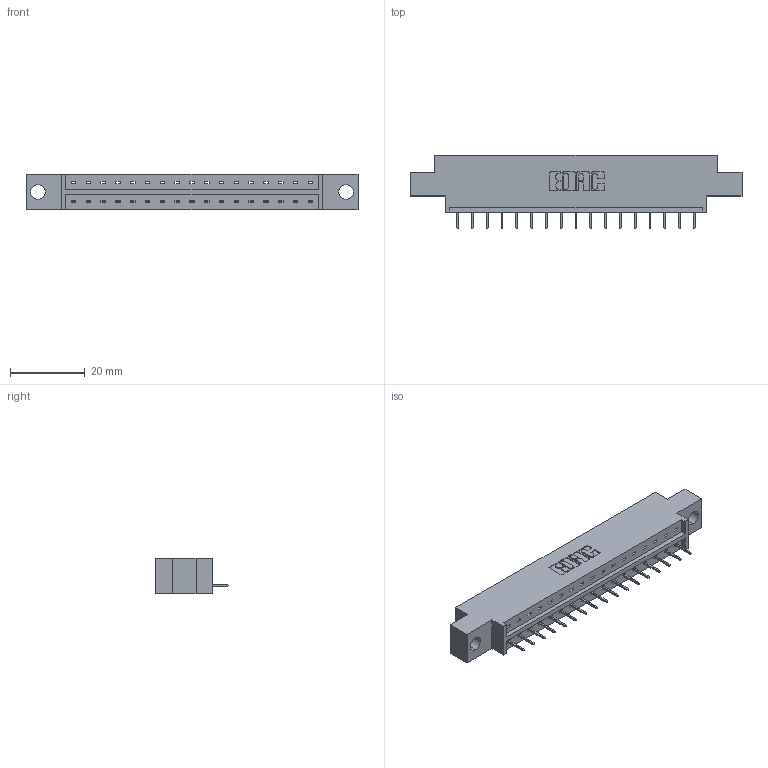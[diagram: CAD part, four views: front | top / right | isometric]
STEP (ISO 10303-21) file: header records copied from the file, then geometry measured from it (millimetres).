
FILE_DESCRIPTION (( 'STEP AP203' ), '1' );
FILE_NAME ('333-017-524-604.STEP', '2019-08-09T11:58:53', ( '' ), ( '' ), 'SwSTEP 2.0', 'SolidWorks 2016', '' );
FILE_SCHEMA (( 'CONFIG_CONTROL_DESIGN' ));
Length unit declared in the file: inch
Products named in the file (3): 333 Part_Offset - .156 Dia - TH; 333-017-524-604; 345-292-001_345-293-124
Assembly tree (18 placements, depth 2):
  333-017-524-604
    333 Part_Offset - .156 Dia - TH
    345-292-001_345-293-124  x17
Bounding box: 88.9 x 19.69 x 9.4 mm (x, y, z)
Volume: 8348 mm3; surface area: 8631.4 mm2
Topology: 18 solids, 18 shells, 1172 faces, 3383 edges, 2186 vertices
Faces by surface type: plane 890, cylinder 282
Entity records: 13835 total; most frequent: CARTESIAN_POINT 2397, ORIENTED_EDGE 2350, DIRECTION 2073, EDGE_CURVE 1175, LINE 1051, VECTOR 1051, VERTEX_POINT 778, AXIS2_PLACEMENT_3D 511
